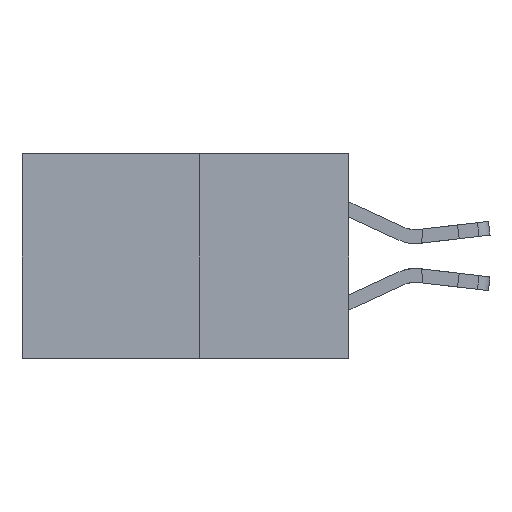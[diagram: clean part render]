
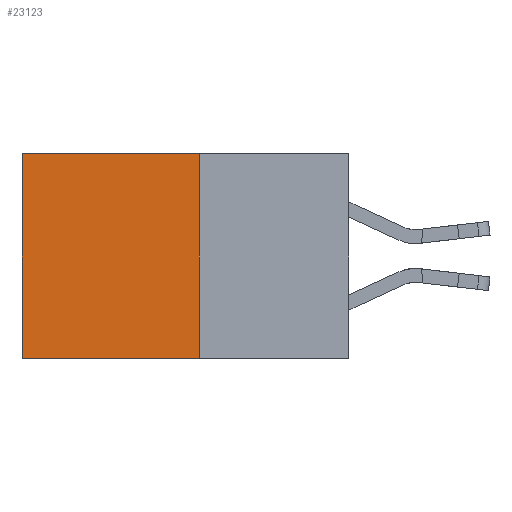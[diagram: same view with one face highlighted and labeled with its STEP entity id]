
A CAD part, left-side view. The second image highlights one B-rep face of the part: STEP entity #23123.
In plain terms, the highlighted planar face has unit normal (-1, 0, 0).
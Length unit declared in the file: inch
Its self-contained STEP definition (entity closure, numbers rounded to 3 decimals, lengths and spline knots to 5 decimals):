
#109 = CARTESIAN_POINT ( 'NONE',  ( 0.277, 0.27, -0.37 ) ) ;
#497 = LINE ( 'NONE', #19776, #11559 ) ;
#1690 = FACE_OUTER_BOUND ( 'NONE', #25758, .T. ) ;
#1798 = AXIS2_PLACEMENT_3D ( 'NONE', #109, #24349, #11213 ) ;
#2239 = VERTEX_POINT ( 'NONE', #13345 ) ;
#2984 = VECTOR ( 'NONE', #16443, 39.37008 ) ;
#3225 = CARTESIAN_POINT ( 'NONE',  ( 0.277, 0.27, 0. ) ) ;
#3569 = DIRECTION ( 'NONE',  ( 0., 0., -1. ) ) ;
#4991 = EDGE_CURVE ( 'NONE', #19483, #2239, #12542, .T. ) ;
#5917 = VECTOR ( 'NONE', #18658, 39.37008 ) ;
#8482 = CARTESIAN_POINT ( 'NONE',  ( 0.277, 0.27, -0.37 ) ) ;
#8634 = CARTESIAN_POINT ( 'NONE',  ( 0.277, 0.27, -0.37 ) ) ;
#8770 = DIRECTION ( 'NONE',  ( 0., 0., -1. ) ) ;
#8981 = PLANE ( 'NONE',  #1798 ) ;
#10142 = CARTESIAN_POINT ( 'NONE',  ( 0.277, 0.27, -0.37 ) ) ;
#10547 = CARTESIAN_POINT ( 'NONE',  ( 0.277, 0.27, 0. ) ) ;
#11213 = DIRECTION ( 'NONE',  ( 0., 0., -1. ) ) ;
#11559 = VECTOR ( 'NONE', #8770, 39.37008 ) ;
#12542 = LINE ( 'NONE', #8634, #5917 ) ;
#13345 = CARTESIAN_POINT ( 'NONE',  ( 0.277, 0.59, -0.37 ) ) ;
#13566 = CARTESIAN_POINT ( 'NONE',  ( 0.277, 0.59, 0. ) ) ;
#13671 = ORIENTED_EDGE ( 'NONE', *, *, #14290, .F. ) ;
#14290 = EDGE_CURVE ( 'NONE', #27359, #19483, #26768, .T. ) ;
#15111 = ORIENTED_EDGE ( 'NONE', *, *, #18348, .T. ) ;
#16443 = DIRECTION ( 'NONE',  ( 0., 1., 0. ) ) ;
#18348 = EDGE_CURVE ( 'NONE', #27359, #24937, #26307, .T. ) ;
#18658 = DIRECTION ( 'NONE',  ( 0., 1., 0. ) ) ;
#19483 = VERTEX_POINT ( 'NONE', #8482 ) ;
#19576 = EDGE_CURVE ( 'NONE', #24937, #2239, #497, .T. ) ;
#19776 = CARTESIAN_POINT ( 'NONE',  ( 0.277, 0.59, -0.37 ) ) ;
#23123 = ADVANCED_FACE ( 'NONE', ( #1690 ), #8981, .F. ) ;
#24003 = ORIENTED_EDGE ( 'NONE', *, *, #19576, .T. ) ;
#24349 = DIRECTION ( 'NONE',  ( 1., 0., 0. ) ) ;
#24937 = VERTEX_POINT ( 'NONE', #13566 ) ;
#25758 = EDGE_LOOP ( 'NONE', ( #24003, #27587, #13671, #15111 ) ) ;
#26111 = VECTOR ( 'NONE', #3569, 39.37008 ) ;
#26307 = LINE ( 'NONE', #3225, #2984 ) ;
#26768 = LINE ( 'NONE', #10142, #26111 ) ;
#27359 = VERTEX_POINT ( 'NONE', #10547 ) ;
#27587 = ORIENTED_EDGE ( 'NONE', *, *, #4991, .F. ) ;
